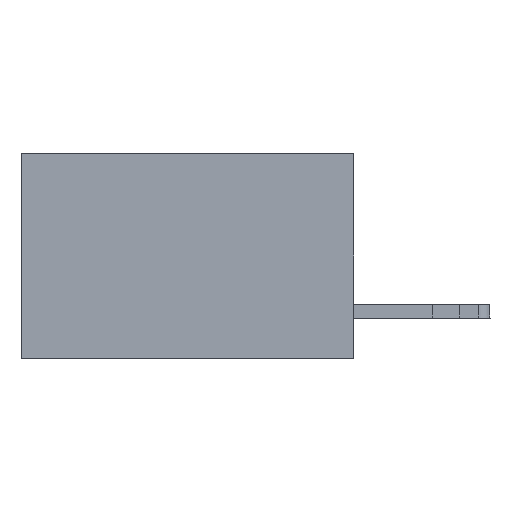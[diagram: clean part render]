
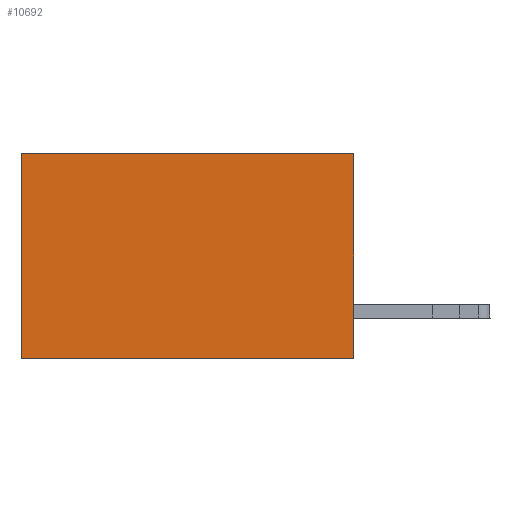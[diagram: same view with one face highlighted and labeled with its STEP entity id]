
A CAD part, left-side view. The second image highlights one B-rep face of the part: STEP entity #10692.
In plain terms, the highlighted planar face has unit normal (-1, 0, 0).
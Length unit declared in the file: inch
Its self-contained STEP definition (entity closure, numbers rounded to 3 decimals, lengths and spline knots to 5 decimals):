
#848 = EDGE_CURVE ( 'NONE', #33089, #3639, #27671, .T. ) ;
#1227 = CARTESIAN_POINT ( 'NONE',  ( 0.2875, 0., 0. ) ) ;
#2221 = AXIS2_PLACEMENT_3D ( 'NONE', #31386, #6322, #25877 ) ;
#2822 = CARTESIAN_POINT ( 'NONE',  ( 0.2875, 0., -0.37 ) ) ;
#3515 = CARTESIAN_POINT ( 'NONE',  ( 0.2875, 0.6, -0.37 ) ) ;
#3639 = VERTEX_POINT ( 'NONE', #3515 ) ;
#4885 = DIRECTION ( 'NONE',  ( 0., 1., 0. ) ) ;
#5343 = VECTOR ( 'NONE', #28262, 39.37008 ) ;
#5694 = LINE ( 'NONE', #9353, #14071 ) ;
#6322 = DIRECTION ( 'NONE',  ( 1., 0., 0. ) ) ;
#8162 = EDGE_LOOP ( 'NONE', ( #18713, #31500, #11507, #28973 ) ) ;
#9353 = CARTESIAN_POINT ( 'NONE',  ( 0.2875, 0., 0. ) ) ;
#10692 = ADVANCED_FACE ( 'NONE', ( #21265 ), #23042, .F. ) ;
#11507 = ORIENTED_EDGE ( 'NONE', *, *, #15139, .F. ) ;
#12050 = DIRECTION ( 'NONE',  ( 0., 1., 0. ) ) ;
#12131 = CARTESIAN_POINT ( 'NONE',  ( 0.2875, 0., 0. ) ) ;
#12524 = LINE ( 'NONE', #12131, #33036 ) ;
#14071 = VECTOR ( 'NONE', #12050, 39.37008 ) ;
#15139 = EDGE_CURVE ( 'NONE', #16399, #28501, #12524, .T. ) ;
#16399 = VERTEX_POINT ( 'NONE', #1227 ) ;
#18713 = ORIENTED_EDGE ( 'NONE', *, *, #848, .T. ) ;
#18750 = LINE ( 'NONE', #21618, #33571 ) ;
#20510 = DIRECTION ( 'NONE',  ( 0., 0., -1. ) ) ;
#20876 = EDGE_CURVE ( 'NONE', #16399, #33089, #5694, .T. ) ;
#21265 = FACE_OUTER_BOUND ( 'NONE', #8162, .T. ) ;
#21618 = CARTESIAN_POINT ( 'NONE',  ( 0.2875, 0., -0.37 ) ) ;
#23042 = PLANE ( 'NONE',  #2221 ) ;
#25877 = DIRECTION ( 'NONE',  ( 0., 0., -1. ) ) ;
#27671 = LINE ( 'NONE', #28567, #5343 ) ;
#28262 = DIRECTION ( 'NONE',  ( 0., 0., -1. ) ) ;
#28501 = VERTEX_POINT ( 'NONE', #2822 ) ;
#28567 = CARTESIAN_POINT ( 'NONE',  ( 0.2875, 0.6, 0. ) ) ;
#28973 = ORIENTED_EDGE ( 'NONE', *, *, #20876, .T. ) ;
#31386 = CARTESIAN_POINT ( 'NONE',  ( 0.2875, 0., 0. ) ) ;
#31500 = ORIENTED_EDGE ( 'NONE', *, *, #35930, .F. ) ;
#31773 = CARTESIAN_POINT ( 'NONE',  ( 0.2875, 0.6, 0. ) ) ;
#33036 = VECTOR ( 'NONE', #20510, 39.37008 ) ;
#33089 = VERTEX_POINT ( 'NONE', #31773 ) ;
#33571 = VECTOR ( 'NONE', #4885, 39.37008 ) ;
#35930 = EDGE_CURVE ( 'NONE', #28501, #3639, #18750, .T. ) ;
